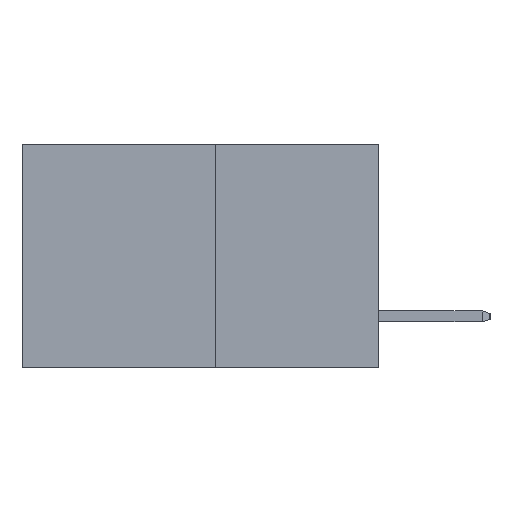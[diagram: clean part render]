
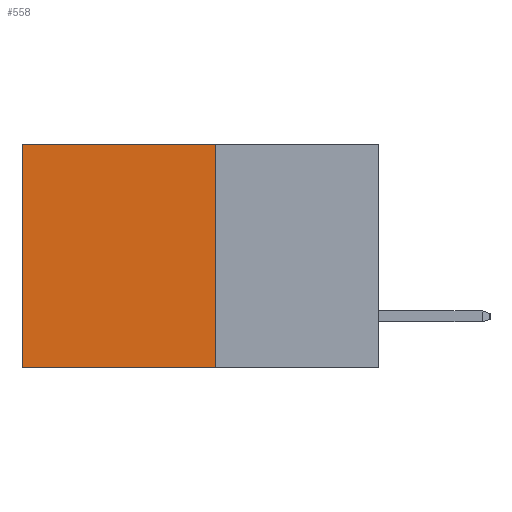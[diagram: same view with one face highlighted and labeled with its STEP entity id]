
A CAD part, left-side view. The second image highlights one B-rep face of the part: STEP entity #558.
In plain terms, the highlighted planar face has unit normal (-1, 0, 0).
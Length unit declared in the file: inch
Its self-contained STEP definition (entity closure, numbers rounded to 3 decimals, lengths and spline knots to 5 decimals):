
#558 = ADVANCED_FACE ( 'NONE', ( #15935 ), #18720, .F. ) ;
#901 = ORIENTED_EDGE ( 'NONE', *, *, #7819, .F. ) ;
#1904 = EDGE_CURVE ( 'NONE', #7906, #11184, #8199, .T. ) ;
#2878 = ORIENTED_EDGE ( 'NONE', *, *, #6803, .T. ) ;
#3778 = CARTESIAN_POINT ( 'NONE',  ( 0.277, 0.59, -0.37 ) ) ;
#3840 = ORIENTED_EDGE ( 'NONE', *, *, #9364, .F. ) ;
#5092 = CARTESIAN_POINT ( 'NONE',  ( 0.277, 0.27, 0. ) ) ;
#6033 = CARTESIAN_POINT ( 'NONE',  ( 0.277, 0.59, 0. ) ) ;
#6803 = EDGE_CURVE ( 'NONE', #11184, #19480, #12518, .T. ) ;
#7819 = EDGE_CURVE ( 'NONE', #7906, #19738, #8630, .T. ) ;
#7906 = VERTEX_POINT ( 'NONE', #5092 ) ;
#8199 = LINE ( 'NONE', #9336, #15878 ) ;
#8439 = VECTOR ( 'NONE', #19428, 39.37008 ) ;
#8630 = LINE ( 'NONE', #17265, #12709 ) ;
#8742 = DIRECTION ( 'NONE',  ( 0., 1., 0. ) ) ;
#9336 = CARTESIAN_POINT ( 'NONE',  ( 0.277, 0.27, 0. ) ) ;
#9364 = EDGE_CURVE ( 'NONE', #19738, #19480, #12185, .T. ) ;
#9616 = DIRECTION ( 'NONE',  ( 0., 0., -1. ) ) ;
#10239 = CARTESIAN_POINT ( 'NONE',  ( 0.277, 0.59, -0.37 ) ) ;
#10494 = CARTESIAN_POINT ( 'NONE',  ( 0.277, 0.27, -0.37 ) ) ;
#10826 = CARTESIAN_POINT ( 'NONE',  ( 0.277, 0.27, -0.37 ) ) ;
#11184 = VERTEX_POINT ( 'NONE', #6033 ) ;
#12185 = LINE ( 'NONE', #10826, #15788 ) ;
#12369 = DIRECTION ( 'NONE',  ( 0., 1., 0. ) ) ;
#12518 = LINE ( 'NONE', #10239, #8439 ) ;
#12709 = VECTOR ( 'NONE', #9616, 39.37008 ) ;
#15335 = ORIENTED_EDGE ( 'NONE', *, *, #1904, .T. ) ;
#15346 = AXIS2_PLACEMENT_3D ( 'NONE', #18566, #17282, #17267 ) ;
#15788 = VECTOR ( 'NONE', #12369, 39.37008 ) ;
#15878 = VECTOR ( 'NONE', #8742, 39.37008 ) ;
#15935 = FACE_OUTER_BOUND ( 'NONE', #18319, .T. ) ;
#17265 = CARTESIAN_POINT ( 'NONE',  ( 0.277, 0.27, -0.37 ) ) ;
#17267 = DIRECTION ( 'NONE',  ( 0., 0., -1. ) ) ;
#17282 = DIRECTION ( 'NONE',  ( 1., 0., 0. ) ) ;
#18319 = EDGE_LOOP ( 'NONE', ( #2878, #3840, #901, #15335 ) ) ;
#18566 = CARTESIAN_POINT ( 'NONE',  ( 0.277, 0.27, -0.37 ) ) ;
#18720 = PLANE ( 'NONE',  #15346 ) ;
#19428 = DIRECTION ( 'NONE',  ( 0., 0., -1. ) ) ;
#19480 = VERTEX_POINT ( 'NONE', #3778 ) ;
#19738 = VERTEX_POINT ( 'NONE', #10494 ) ;
